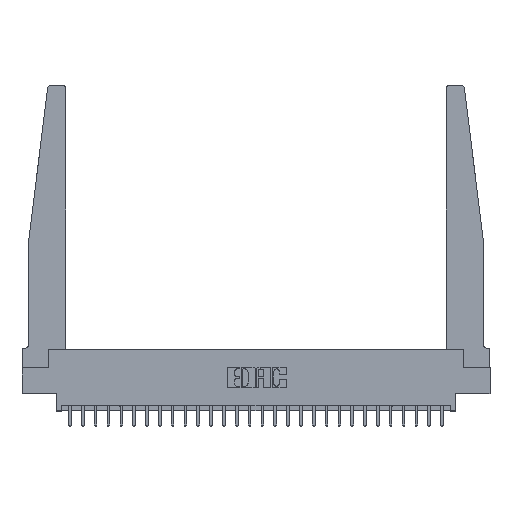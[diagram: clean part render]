
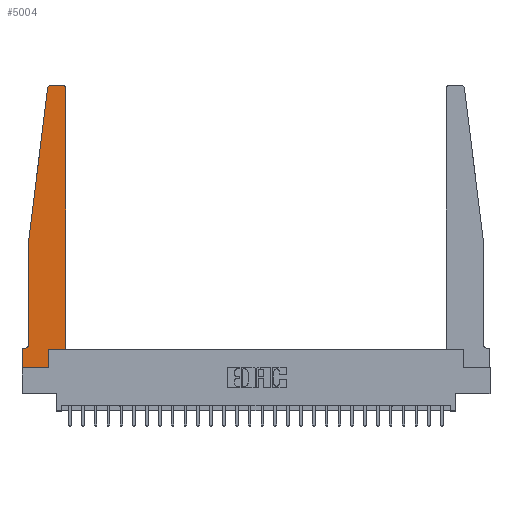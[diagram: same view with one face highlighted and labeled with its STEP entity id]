
A CAD part, top view. The second image highlights one B-rep face of the part: STEP entity #5004.
In plain terms, the highlighted planar face has unit normal (0, 0, 1).
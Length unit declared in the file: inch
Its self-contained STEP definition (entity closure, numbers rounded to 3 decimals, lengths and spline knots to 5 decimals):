
#196 = DIRECTION ( 'NONE',  ( 1., 0., 0. ) ) ;
#565 = VECTOR ( 'NONE', #196, 39.37008 ) ;
#593 = VECTOR ( 'NONE', #17538, 39.37008 ) ;
#1163 = LINE ( 'NONE', #9314, #593 ) ;
#1270 = EDGE_CURVE ( 'NONE', #1785, #10541, #19553, .T. ) ;
#1677 = CARTESIAN_POINT ( 'NONE',  ( 0.25, 2.75, 0.37 ) ) ;
#1785 = VERTEX_POINT ( 'NONE', #20188 ) ;
#1880 = DIRECTION ( 'NONE',  ( 0., 1., 0. ) ) ;
#1881 = CARTESIAN_POINT ( 'NONE',  ( 0.27653, 2.75, 0.37 ) ) ;
#1992 = ORIENTED_EDGE ( 'NONE', *, *, #1270, .T. ) ;
#2379 = ORIENTED_EDGE ( 'NONE', *, *, #22321, .T. ) ;
#2608 = CARTESIAN_POINT ( 'NONE',  ( 0.065, 0.2375, 0.37 ) ) ;
#3392 = DIRECTION ( 'NONE',  ( 0., -1., 0. ) ) ;
#3883 = CARTESIAN_POINT ( 'NONE',  ( 0., 0., 0.37 ) ) ;
#4328 = CARTESIAN_POINT ( 'NONE',  ( 0., 0., 0.37 ) ) ;
#4565 = PLANE ( 'NONE',  #15267 ) ;
#4985 = ORIENTED_EDGE ( 'NONE', *, *, #23954, .T. ) ;
#5004 = ADVANCED_FACE ( 'NONE', ( #14653 ), #4565, .T. ) ;
#5430 = EDGE_CURVE ( 'NONE', #21952, #9688, #19518, .T. ) ;
#5451 = CARTESIAN_POINT ( 'NONE',  ( 0.015, 0.2375, 0.37 ) ) ;
#6801 = EDGE_CURVE ( 'NONE', #24426, #14104, #15974, .T. ) ;
#7724 = DIRECTION ( 'NONE',  ( 0., 0., -1. ) ) ;
#8015 = AXIS2_PLACEMENT_3D ( 'NONE', #9224, #15426, #17438 ) ;
#8019 = LINE ( 'NONE', #24064, #23952 ) ;
#8355 = DIRECTION ( 'NONE',  ( 0., 1., 0. ) ) ;
#8365 = EDGE_CURVE ( 'NONE', #9688, #1785, #11009, .T. ) ;
#8481 = ORIENTED_EDGE ( 'NONE', *, *, #14772, .T. ) ;
#8682 = VECTOR ( 'NONE', #23748, 39.37008 ) ;
#8926 = CARTESIAN_POINT ( 'NONE',  ( 0., 0.1875, 0.37 ) ) ;
#9007 = CARTESIAN_POINT ( 'NONE',  ( 0.2605, 0.18, 0.37 ) ) ;
#9224 = CARTESIAN_POINT ( 'NONE',  ( 0.395, 2.72, 0.37 ) ) ;
#9314 = CARTESIAN_POINT ( 'NONE',  ( 0.065, 0.1875, 0.37 ) ) ;
#9506 = EDGE_CURVE ( 'NONE', #14104, #15898, #14164, .T. ) ;
#9688 = VERTEX_POINT ( 'NONE', #16803 ) ;
#9861 = EDGE_LOOP ( 'NONE', ( #23221, #11390, #12783, #1992, #2379, #20561, #13511, #21205, #13653, #17772, #8481, #4985 ) ) ;
#10359 = CARTESIAN_POINT ( 'NONE',  ( 0.395, 2.75, 0.37 ) ) ;
#10499 = LINE ( 'NONE', #16410, #12126 ) ;
#10541 = VERTEX_POINT ( 'NONE', #2608 ) ;
#10775 = EDGE_CURVE ( 'NONE', #26464, #21952, #15744, .T. ) ;
#11009 = LINE ( 'NONE', #25829, #21056 ) ;
#11390 = ORIENTED_EDGE ( 'NONE', *, *, #5430, .T. ) ;
#11538 = DIRECTION ( 'NONE',  ( -0.122, -0.992, 0. ) ) ;
#12011 = CARTESIAN_POINT ( 'NONE',  ( 0.2605, 0., 0.37 ) ) ;
#12114 = VERTEX_POINT ( 'NONE', #14156 ) ;
#12126 = VECTOR ( 'NONE', #8355, 39.37008 ) ;
#12650 = AXIS2_PLACEMENT_3D ( 'NONE', #21058, #23521, #25275 ) ;
#12783 = ORIENTED_EDGE ( 'NONE', *, *, #8365, .T. ) ;
#13425 = VERTEX_POINT ( 'NONE', #21248 ) ;
#13511 = ORIENTED_EDGE ( 'NONE', *, *, #6801, .T. ) ;
#13627 = VECTOR ( 'NONE', #15997, 39.37008 ) ;
#13653 = ORIENTED_EDGE ( 'NONE', *, *, #24092, .T. ) ;
#13954 = VECTOR ( 'NONE', #18277, 39.37008 ) ;
#14104 = VERTEX_POINT ( 'NONE', #3883 ) ;
#14156 = CARTESIAN_POINT ( 'NONE',  ( 0.425, 2.72, 0.37 ) ) ;
#14164 = LINE ( 'NONE', #4328, #565 ) ;
#14653 = FACE_OUTER_BOUND ( 'NONE', #9861, .T. ) ;
#14772 = EDGE_CURVE ( 'NONE', #17742, #12114, #10499, .T. ) ;
#15194 = DIRECTION ( 'NONE',  ( 1., 0., 0. ) ) ;
#15267 = AXIS2_PLACEMENT_3D ( 'NONE', #17189, #15327, #15194 ) ;
#15327 = DIRECTION ( 'NONE',  ( 0., 0., 1. ) ) ;
#15386 = CARTESIAN_POINT ( 'NONE',  ( 0.425, 0.18, 0.37 ) ) ;
#15426 = DIRECTION ( 'NONE',  ( 0., 0., 1. ) ) ;
#15721 = CIRCLE ( 'NONE', #8015, 0.03 ) ;
#15744 = LINE ( 'NONE', #1677, #13627 ) ;
#15898 = VERTEX_POINT ( 'NONE', #12011 ) ;
#15968 = LINE ( 'NONE', #18130, #13954 ) ;
#15974 = LINE ( 'NONE', #19909, #20235 ) ;
#15997 = DIRECTION ( 'NONE',  ( -1., 0., 0. ) ) ;
#16304 = VERTEX_POINT ( 'NONE', #9007 ) ;
#16410 = CARTESIAN_POINT ( 'NONE',  ( 0.425, 0.18, 0.37 ) ) ;
#16803 = CARTESIAN_POINT ( 'NONE',  ( 0.24675, 2.72367, 0.37 ) ) ;
#17189 = CARTESIAN_POINT ( 'NONE',  ( 0., 0.1875, 0.37 ) ) ;
#17438 = DIRECTION ( 'NONE',  ( 1., 0., 0. ) ) ;
#17537 = CARTESIAN_POINT ( 'NONE',  ( 0.065, 1.25, 0.37 ) ) ;
#17538 = DIRECTION ( 'NONE',  ( -1., 0., 0. ) ) ;
#17553 = DIRECTION ( 'NONE',  ( -1., 0., 0. ) ) ;
#17742 = VERTEX_POINT ( 'NONE', #15386 ) ;
#17766 = EDGE_CURVE ( 'NONE', #13425, #24426, #1163, .T. ) ;
#17772 = ORIENTED_EDGE ( 'NONE', *, *, #21389, .T. ) ;
#18130 = CARTESIAN_POINT ( 'NONE',  ( 0.425, 0.18, 0.37 ) ) ;
#18269 = AXIS2_PLACEMENT_3D ( 'NONE', #5451, #7724, #17553 ) ;
#18277 = DIRECTION ( 'NONE',  ( 1., 0., 0. ) ) ;
#19518 = CIRCLE ( 'NONE', #12650, 0.03 ) ;
#19553 = LINE ( 'NONE', #17537, #8682 ) ;
#19909 = CARTESIAN_POINT ( 'NONE',  ( 0., 0., 0.37 ) ) ;
#20188 = CARTESIAN_POINT ( 'NONE',  ( 0.065, 1.25, 0.37 ) ) ;
#20235 = VECTOR ( 'NONE', #3392, 39.37008 ) ;
#20561 = ORIENTED_EDGE ( 'NONE', *, *, #17766, .T. ) ;
#21056 = VECTOR ( 'NONE', #11538, 39.37008 ) ;
#21058 = CARTESIAN_POINT ( 'NONE',  ( 0.27653, 2.72, 0.37 ) ) ;
#21205 = ORIENTED_EDGE ( 'NONE', *, *, #9506, .T. ) ;
#21248 = CARTESIAN_POINT ( 'NONE',  ( 0.015, 0.1875, 0.37 ) ) ;
#21389 = EDGE_CURVE ( 'NONE', #16304, #17742, #15968, .T. ) ;
#21952 = VERTEX_POINT ( 'NONE', #1881 ) ;
#22321 = EDGE_CURVE ( 'NONE', #10541, #13425, #25174, .T. ) ;
#23221 = ORIENTED_EDGE ( 'NONE', *, *, #10775, .T. ) ;
#23521 = DIRECTION ( 'NONE',  ( 0., 0., 1. ) ) ;
#23748 = DIRECTION ( 'NONE',  ( 0., -1., 0. ) ) ;
#23952 = VECTOR ( 'NONE', #1880, 39.37008 ) ;
#23954 = EDGE_CURVE ( 'NONE', #12114, #26464, #15721, .T. ) ;
#24064 = CARTESIAN_POINT ( 'NONE',  ( 0.2605, 0.18, 0.37 ) ) ;
#24092 = EDGE_CURVE ( 'NONE', #15898, #16304, #8019, .T. ) ;
#24426 = VERTEX_POINT ( 'NONE', #8926 ) ;
#25174 = CIRCLE ( 'NONE', #18269, 0.05 ) ;
#25275 = DIRECTION ( 'NONE',  ( 1., 0., 0. ) ) ;
#25829 = CARTESIAN_POINT ( 'NONE',  ( 0.065, 1.25, 0.37 ) ) ;
#26464 = VERTEX_POINT ( 'NONE', #10359 ) ;
